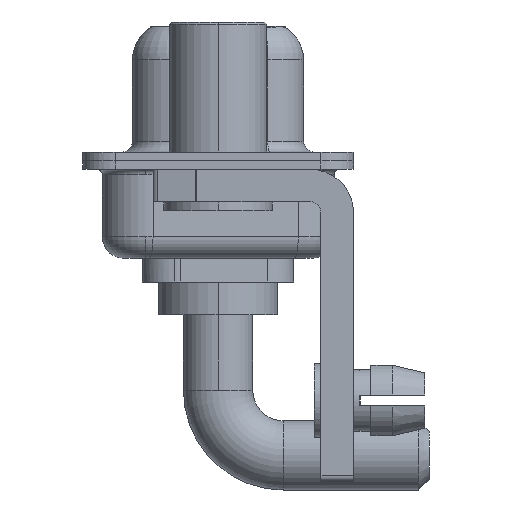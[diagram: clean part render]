
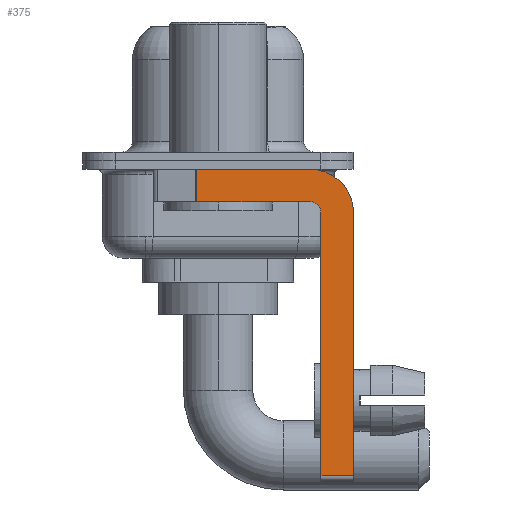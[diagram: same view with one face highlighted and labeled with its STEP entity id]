
A CAD part, left-side view. The second image highlights one B-rep face of the part: STEP entity #375.
In plain terms, the highlighted planar face has unit normal (-1, 0, 0).
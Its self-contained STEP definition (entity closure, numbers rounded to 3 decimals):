
#35 = EDGE_CURVE ( 'NONE', #3436, #15756, #2406, .T. ) ;
#375 = ADVANCED_FACE ( 'NONE', ( #5908 ), #13709, .F. ) ;
#1281 = VERTEX_POINT ( 'NONE', #9884 ) ;
#1372 = ORIENTED_EDGE ( 'NONE', *, *, #35, .F. ) ;
#1442 = LINE ( 'NONE', #5064, #13670 ) ;
#2112 = DIRECTION ( 'NONE',  ( 0., -1., 0. ) ) ;
#2138 = CARTESIAN_POINT ( 'NONE',  ( -2.9, 0.978, -0.4 ) ) ;
#2406 = LINE ( 'NONE', #11508, #9666 ) ;
#2567 = AXIS2_PLACEMENT_3D ( 'NONE', #5835, #3185, #7097 ) ;
#3185 = DIRECTION ( 'NONE',  ( -1., 0., 0. ) ) ;
#3436 = VERTEX_POINT ( 'NONE', #9759 ) ;
#3909 = VERTEX_POINT ( 'NONE', #2138 ) ;
#3911 = LINE ( 'NONE', #12772, #13474 ) ;
#3947 = DIRECTION ( 'NONE',  ( 1., 0., 0. ) ) ;
#3995 = CARTESIAN_POINT ( 'NONE',  ( -2.9, -4.25, -1.9 ) ) ;
#4519 = DIRECTION ( 'NONE',  ( 1., 0., 0. ) ) ;
#4528 = EDGE_LOOP ( 'NONE', ( #6047, #15720, #9770, #15233, #1372, #7108, #11860, #10842 ) ) ;
#5064 = CARTESIAN_POINT ( 'NONE',  ( -2.9, 3., -0.4 ) ) ;
#5150 = DIRECTION ( 'NONE',  ( 0., 0., -1. ) ) ;
#5189 = EDGE_CURVE ( 'NONE', #15756, #1281, #6385, .T. ) ;
#5194 = DIRECTION ( 'NONE',  ( 0., 1., 0. ) ) ;
#5207 = CARTESIAN_POINT ( 'NONE',  ( -2.9, -4.75, -2.4 ) ) ;
#5552 = VECTOR ( 'NONE', #2112, 1000. ) ;
#5729 = DIRECTION ( 'NONE',  ( 0., 0., -1. ) ) ;
#5835 = CARTESIAN_POINT ( 'NONE',  ( -2.9, -4.25, -2.4 ) ) ;
#5908 = FACE_OUTER_BOUND ( 'NONE', #4528, .T. ) ;
#6032 = LINE ( 'NONE', #9858, #5552 ) ;
#6047 = ORIENTED_EDGE ( 'NONE', *, *, #7841, .F. ) ;
#6098 = VERTEX_POINT ( 'NONE', #8112 ) ;
#6385 = CIRCLE ( 'NONE', #2567, 0.5 ) ;
#6393 = EDGE_CURVE ( 'NONE', #1281, #15038, #10384, .T. ) ;
#6424 = EDGE_CURVE ( 'NONE', #6098, #9649, #3911, .T. ) ;
#6624 = EDGE_CURVE ( 'NONE', #3909, #15038, #9269, .T. ) ;
#7097 = DIRECTION ( 'NONE',  ( 0., 0., 1. ) ) ;
#7108 = ORIENTED_EDGE ( 'NONE', *, *, #11575, .T. ) ;
#7189 = AXIS2_PLACEMENT_3D ( 'NONE', #10590, #3947, #5150 ) ;
#7841 = EDGE_CURVE ( 'NONE', #3909, #8520, #1442, .T. ) ;
#7911 = DIRECTION ( 'NONE',  ( 0., 0., -1. ) ) ;
#8112 = CARTESIAN_POINT ( 'NONE',  ( -2.9, -6.25, -2.4 ) ) ;
#8520 = VERTEX_POINT ( 'NONE', #16234 ) ;
#8821 = CARTESIAN_POINT ( 'NONE',  ( -2.9, -6.25, -14.55 ) ) ;
#8880 = VECTOR ( 'NONE', #13190, 1000. ) ;
#9269 = LINE ( 'NONE', #14433, #8880 ) ;
#9649 = VERTEX_POINT ( 'NONE', #8821 ) ;
#9666 = VECTOR ( 'NONE', #16685, 1000. ) ;
#9759 = CARTESIAN_POINT ( 'NONE',  ( -2.9, -4.75, -14.55 ) ) ;
#9770 = ORIENTED_EDGE ( 'NONE', *, *, #6393, .F. ) ;
#9858 = CARTESIAN_POINT ( 'NONE',  ( -2.9, -4.25, -14.55 ) ) ;
#9884 = CARTESIAN_POINT ( 'NONE',  ( -2.9, -4.25, -1.9 ) ) ;
#10384 = LINE ( 'NONE', #3995, #12126 ) ;
#10590 = CARTESIAN_POINT ( 'NONE',  ( -2.9, -4.25, -2.4 ) ) ;
#10787 = AXIS2_PLACEMENT_3D ( 'NONE', #13532, #4519, #5729 ) ;
#10842 = ORIENTED_EDGE ( 'NONE', *, *, #16768, .F. ) ;
#11508 = CARTESIAN_POINT ( 'NONE',  ( -2.9, -4.75, -14.8 ) ) ;
#11575 = EDGE_CURVE ( 'NONE', #3436, #9649, #6032, .T. ) ;
#11680 = CARTESIAN_POINT ( 'NONE',  ( -2.9, 0.978, -1.9 ) ) ;
#11860 = ORIENTED_EDGE ( 'NONE', *, *, #6424, .F. ) ;
#12000 = DIRECTION ( 'NONE',  ( 0., -1., 0. ) ) ;
#12126 = VECTOR ( 'NONE', #5194, 1000. ) ;
#12772 = CARTESIAN_POINT ( 'NONE',  ( -2.9, -6.25, -2.4 ) ) ;
#13190 = DIRECTION ( 'NONE',  ( 0., 0., -1. ) ) ;
#13474 = VECTOR ( 'NONE', #7911, 1000. ) ;
#13532 = CARTESIAN_POINT ( 'NONE',  ( -2.9, -4.25, -2.4 ) ) ;
#13670 = VECTOR ( 'NONE', #12000, 1000. ) ;
#13709 = PLANE ( 'NONE',  #10787 ) ;
#14433 = CARTESIAN_POINT ( 'NONE',  ( -2.9, 0.978, -1.9 ) ) ;
#15038 = VERTEX_POINT ( 'NONE', #11680 ) ;
#15233 = ORIENTED_EDGE ( 'NONE', *, *, #5189, .F. ) ;
#15720 = ORIENTED_EDGE ( 'NONE', *, *, #6624, .T. ) ;
#15756 = VERTEX_POINT ( 'NONE', #5207 ) ;
#15858 = CIRCLE ( 'NONE', #7189, 2. ) ;
#16234 = CARTESIAN_POINT ( 'NONE',  ( -2.9, -4.25, -0.4 ) ) ;
#16685 = DIRECTION ( 'NONE',  ( 0., 0., 1. ) ) ;
#16768 = EDGE_CURVE ( 'NONE', #8520, #6098, #15858, .T. ) ;
